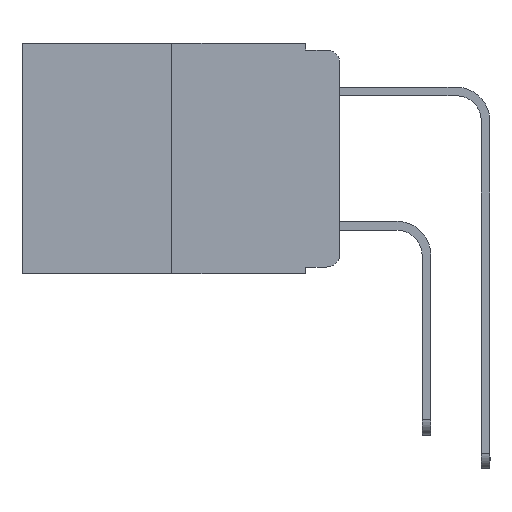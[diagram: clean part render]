
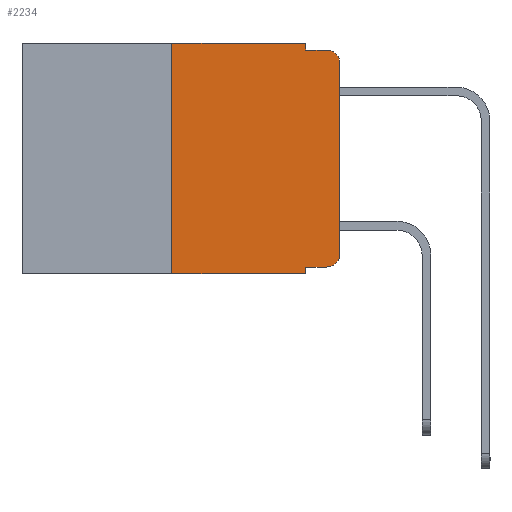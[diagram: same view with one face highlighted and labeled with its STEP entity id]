
A CAD part, left-side view. The second image highlights one B-rep face of the part: STEP entity #2234.
In plain terms, the highlighted planar face has unit normal (-1, 0, 0).
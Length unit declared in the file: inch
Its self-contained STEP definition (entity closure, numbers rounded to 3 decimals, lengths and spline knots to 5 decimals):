
#400 = CARTESIAN_POINT ( 'NONE',  ( 0., 0.473, 0. ) ) ;
#720 = CARTESIAN_POINT ( 'NONE',  ( 0., 0.051, -0.343 ) ) ;
#731 = LINE ( 'NONE', #4260, #15191 ) ;
#951 = VECTOR ( 'NONE', #11827, 39.37008 ) ;
#984 = CARTESIAN_POINT ( 'NONE',  ( 0., 0.02, -0.03 ) ) ;
#1032 = EDGE_CURVE ( 'NONE', #10891, #14518, #7354, .T. ) ;
#1217 = ORIENTED_EDGE ( 'NONE', *, *, #13972, .T. ) ;
#1362 = CIRCLE ( 'NONE', #10044, 0.02 ) ;
#1493 = VERTEX_POINT ( 'NONE', #15753 ) ;
#1634 = CARTESIAN_POINT ( 'NONE',  ( 0., 0.051, 0. ) ) ;
#2210 = DIRECTION ( 'NONE',  ( 0., -1., 0. ) ) ;
#2234 = ADVANCED_FACE ( 'NONE', ( #4588 ), #14359, .F. ) ;
#2250 = DIRECTION ( 'NONE',  ( 0., 0., -1. ) ) ;
#2349 = ORIENTED_EDGE ( 'NONE', *, *, #10252, .T. ) ;
#3374 = CARTESIAN_POINT ( 'NONE',  ( 0., 0.473, 0. ) ) ;
#3436 = VERTEX_POINT ( 'NONE', #7464 ) ;
#3520 = EDGE_CURVE ( 'NONE', #14518, #13787, #6742, .T. ) ;
#3667 = CIRCLE ( 'NONE', #12609, 0.02 ) ;
#3773 = DIRECTION ( 'NONE',  ( 0., 0., -1. ) ) ;
#4206 = EDGE_CURVE ( 'NONE', #8390, #3436, #11022, .T. ) ;
#4260 = CARTESIAN_POINT ( 'NONE',  ( 0., 0.473, -0.343 ) ) ;
#4335 = VECTOR ( 'NONE', #5802, 39.37008 ) ;
#4362 = LINE ( 'NONE', #4530, #4335 ) ;
#4530 = CARTESIAN_POINT ( 'NONE',  ( 0., 0.25, 0. ) ) ;
#4588 = FACE_OUTER_BOUND ( 'NONE', #11915, .T. ) ;
#5110 = CARTESIAN_POINT ( 'NONE',  ( 0., 0.051, 0. ) ) ;
#5346 = VECTOR ( 'NONE', #11691, 39.37008 ) ;
#5802 = DIRECTION ( 'NONE',  ( 0., 0., 1. ) ) ;
#5816 = CARTESIAN_POINT ( 'NONE',  ( 0., 0.051, -0.333 ) ) ;
#5854 = DIRECTION ( 'NONE',  ( 1., 0., 0. ) ) ;
#5883 = ORIENTED_EDGE ( 'NONE', *, *, #10617, .F. ) ;
#6068 = CARTESIAN_POINT ( 'NONE',  ( 0., 0., -0.313 ) ) ;
#6180 = VECTOR ( 'NONE', #8741, 39.37008 ) ;
#6183 = CARTESIAN_POINT ( 'NONE',  ( 0., 0.051, 0. ) ) ;
#6381 = ORIENTED_EDGE ( 'NONE', *, *, #14157, .T. ) ;
#6414 = CARTESIAN_POINT ( 'NONE',  ( 0., 0.02, -0.01 ) ) ;
#6742 = LINE ( 'NONE', #11635, #12632 ) ;
#6800 = LINE ( 'NONE', #400, #5346 ) ;
#6941 = CARTESIAN_POINT ( 'NONE',  ( 0., 0., 0. ) ) ;
#7234 = AXIS2_PLACEMENT_3D ( 'NONE', #3374, #5854, #2250 ) ;
#7354 = LINE ( 'NONE', #5110, #7685 ) ;
#7464 = CARTESIAN_POINT ( 'NONE',  ( 0., 0.02, -0.333 ) ) ;
#7685 = VECTOR ( 'NONE', #14972, 39.37008 ) ;
#7795 = DIRECTION ( 'NONE',  ( 0., -1., 0. ) ) ;
#8164 = CARTESIAN_POINT ( 'NONE',  ( 0., 0.051, -0.01 ) ) ;
#8339 = EDGE_CURVE ( 'NONE', #8818, #10891, #6800, .T. ) ;
#8340 = VERTEX_POINT ( 'NONE', #720 ) ;
#8390 = VERTEX_POINT ( 'NONE', #14259 ) ;
#8535 = CARTESIAN_POINT ( 'NONE',  ( 0., 0., -0.03 ) ) ;
#8741 = DIRECTION ( 'NONE',  ( 0., 0., -1. ) ) ;
#8818 = VERTEX_POINT ( 'NONE', #9410 ) ;
#9410 = CARTESIAN_POINT ( 'NONE',  ( 0., 0.25, 0. ) ) ;
#9480 = ORIENTED_EDGE ( 'NONE', *, *, #15446, .T. ) ;
#9537 = VERTEX_POINT ( 'NONE', #8535 ) ;
#10044 = AXIS2_PLACEMENT_3D ( 'NONE', #10150, #13934, #14988 ) ;
#10150 = CARTESIAN_POINT ( 'NONE',  ( 0., 0.02, -0.313 ) ) ;
#10252 = EDGE_CURVE ( 'NONE', #14676, #9537, #15447, .T. ) ;
#10465 = ORIENTED_EDGE ( 'NONE', *, *, #12461, .F. ) ;
#10617 = EDGE_CURVE ( 'NONE', #1493, #8818, #4362, .T. ) ;
#10891 = VERTEX_POINT ( 'NONE', #1634 ) ;
#11022 = LINE ( 'NONE', #5816, #12418 ) ;
#11635 = CARTESIAN_POINT ( 'NONE',  ( 0., 0.051, -0.01 ) ) ;
#11691 = DIRECTION ( 'NONE',  ( 0., -1., 0. ) ) ;
#11827 = DIRECTION ( 'NONE',  ( 0., 0., 1. ) ) ;
#11915 = EDGE_LOOP ( 'NONE', ( #2349, #6381, #15371, #14714, #15724, #5883, #1217, #10465, #12039, #9480 ) ) ;
#12039 = ORIENTED_EDGE ( 'NONE', *, *, #4206, .T. ) ;
#12350 = LINE ( 'NONE', #6183, #6180 ) ;
#12418 = VECTOR ( 'NONE', #2210, 39.37008 ) ;
#12461 = EDGE_CURVE ( 'NONE', #8390, #8340, #12350, .T. ) ;
#12609 = AXIS2_PLACEMENT_3D ( 'NONE', #984, #13225, #3773 ) ;
#12632 = VECTOR ( 'NONE', #15321, 39.37008 ) ;
#13225 = DIRECTION ( 'NONE',  ( -1., 0., 0. ) ) ;
#13787 = VERTEX_POINT ( 'NONE', #6414 ) ;
#13934 = DIRECTION ( 'NONE',  ( -1., 0., 0. ) ) ;
#13972 = EDGE_CURVE ( 'NONE', #1493, #8340, #731, .T. ) ;
#14157 = EDGE_CURVE ( 'NONE', #9537, #13787, #3667, .T. ) ;
#14259 = CARTESIAN_POINT ( 'NONE',  ( 0., 0.051, -0.333 ) ) ;
#14359 = PLANE ( 'NONE',  #7234 ) ;
#14518 = VERTEX_POINT ( 'NONE', #8164 ) ;
#14676 = VERTEX_POINT ( 'NONE', #6068 ) ;
#14714 = ORIENTED_EDGE ( 'NONE', *, *, #1032, .F. ) ;
#14972 = DIRECTION ( 'NONE',  ( 0., 0., -1. ) ) ;
#14988 = DIRECTION ( 'NONE',  ( 0., 0., -1. ) ) ;
#15191 = VECTOR ( 'NONE', #7795, 39.37008 ) ;
#15321 = DIRECTION ( 'NONE',  ( 0., -1., 0. ) ) ;
#15371 = ORIENTED_EDGE ( 'NONE', *, *, #3520, .F. ) ;
#15446 = EDGE_CURVE ( 'NONE', #3436, #14676, #1362, .T. ) ;
#15447 = LINE ( 'NONE', #6941, #951 ) ;
#15724 = ORIENTED_EDGE ( 'NONE', *, *, #8339, .F. ) ;
#15753 = CARTESIAN_POINT ( 'NONE',  ( 0., 0.25, -0.343 ) ) ;
